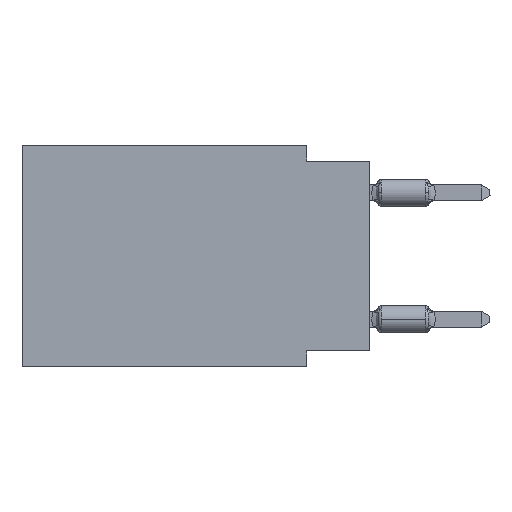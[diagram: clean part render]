
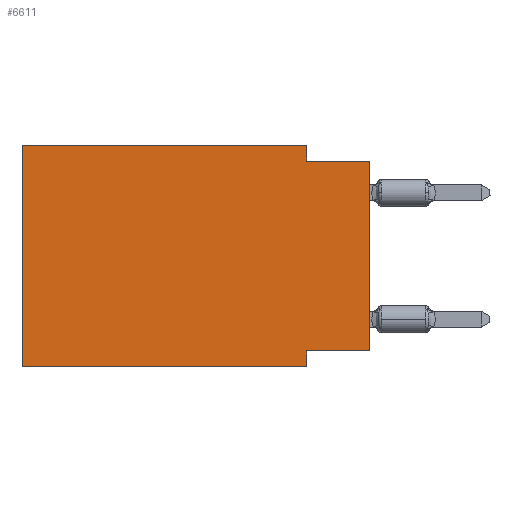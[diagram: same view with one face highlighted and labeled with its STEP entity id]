
A CAD part, left-side view. The second image highlights one B-rep face of the part: STEP entity #6611.
In plain terms, the highlighted planar face has unit normal (-1, 0, 0).
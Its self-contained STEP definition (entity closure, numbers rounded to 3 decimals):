
#25 = VECTOR ( 'NONE', #5033, 1000. ) ;
#152 = ORIENTED_EDGE ( 'NONE', *, *, #23666, .F. ) ;
#1148 = CARTESIAN_POINT ( 'NONE',  ( 0., 13.97, 0. ) ) ;
#2047 = CARTESIAN_POINT ( 'NONE',  ( 0., 13.97, -8.89 ) ) ;
#2530 = ORIENTED_EDGE ( 'NONE', *, *, #20713, .T. ) ;
#3022 = VERTEX_POINT ( 'NONE', #24234 ) ;
#4364 = EDGE_LOOP ( 'NONE', ( #2530, #10978, #5514, #17038, #152, #25755, #10705, #10744 ) ) ;
#4492 = CARTESIAN_POINT ( 'NONE',  ( 0., 13.97, 0. ) ) ;
#4743 = VERTEX_POINT ( 'NONE', #25854 ) ;
#4874 = VERTEX_POINT ( 'NONE', #2047 ) ;
#4876 = EDGE_CURVE ( 'NONE', #5937, #13253, #10589, .T. ) ;
#5033 = DIRECTION ( 'NONE',  ( 0., 0., 1. ) ) ;
#5514 = ORIENTED_EDGE ( 'NONE', *, *, #19162, .F. ) ;
#5937 = VERTEX_POINT ( 'NONE', #9729 ) ;
#6396 = VERTEX_POINT ( 'NONE', #25724 ) ;
#6611 = ADVANCED_FACE ( 'NONE', ( #18299 ), #14349, .F. ) ;
#7750 = EDGE_CURVE ( 'NONE', #8501, #6396, #24331, .T. ) ;
#8501 = VERTEX_POINT ( 'NONE', #12632 ) ;
#9103 = CARTESIAN_POINT ( 'NONE',  ( 0., 0., 0. ) ) ;
#9175 = CARTESIAN_POINT ( 'NONE',  ( 0., 2.54, -8.255 ) ) ;
#9729 = CARTESIAN_POINT ( 'NONE',  ( 0., 0., -8.255 ) ) ;
#10153 = DIRECTION ( 'NONE',  ( 0., 0., -1. ) ) ;
#10405 = DIRECTION ( 'NONE',  ( 0., -1., 0. ) ) ;
#10589 = LINE ( 'NONE', #21653, #26230 ) ;
#10705 = ORIENTED_EDGE ( 'NONE', *, *, #14092, .F. ) ;
#10744 = ORIENTED_EDGE ( 'NONE', *, *, #4876, .F. ) ;
#10776 = DIRECTION ( 'NONE',  ( 0., -1., 0. ) ) ;
#10978 = ORIENTED_EDGE ( 'NONE', *, *, #7750, .F. ) ;
#12194 = EDGE_CURVE ( 'NONE', #4743, #3022, #23680, .T. ) ;
#12384 = CARTESIAN_POINT ( 'NONE',  ( 0., 13.97, 0. ) ) ;
#12632 = CARTESIAN_POINT ( 'NONE',  ( 0., 2.54, -0.635 ) ) ;
#13253 = VERTEX_POINT ( 'NONE', #9175 ) ;
#13336 = VECTOR ( 'NONE', #17233, 1000. ) ;
#13892 = DIRECTION ( 'NONE',  ( 0., 0., 1. ) ) ;
#14092 = EDGE_CURVE ( 'NONE', #13253, #20812, #17506, .T. ) ;
#14349 = PLANE ( 'NONE',  #15550 ) ;
#15550 = AXIS2_PLACEMENT_3D ( 'NONE', #12384, #18711, #10153 ) ;
#17038 = ORIENTED_EDGE ( 'NONE', *, *, #12194, .F. ) ;
#17233 = DIRECTION ( 'NONE',  ( 0., 0., -1. ) ) ;
#17506 = LINE ( 'NONE', #17938, #19445 ) ;
#17897 = DIRECTION ( 'NONE',  ( 0., -1., 0. ) ) ;
#17938 = CARTESIAN_POINT ( 'NONE',  ( 0., 2.54, -8.89 ) ) ;
#18299 = FACE_OUTER_BOUND ( 'NONE', #4364, .T. ) ;
#18711 = DIRECTION ( 'NONE',  ( 1., 0., 0. ) ) ;
#19147 = DIRECTION ( 'NONE',  ( 0., 1., 0. ) ) ;
#19162 = EDGE_CURVE ( 'NONE', #3022, #8501, #21179, .T. ) ;
#19445 = VECTOR ( 'NONE', #19899, 1000. ) ;
#19893 = LINE ( 'NONE', #9103, #25 ) ;
#19899 = DIRECTION ( 'NONE',  ( 0., 0., -1. ) ) ;
#20086 = LINE ( 'NONE', #1148, #24801 ) ;
#20713 = EDGE_CURVE ( 'NONE', #5937, #6396, #19893, .T. ) ;
#20812 = VERTEX_POINT ( 'NONE', #21855 ) ;
#20934 = CARTESIAN_POINT ( 'NONE',  ( 0., 13.97, -8.89 ) ) ;
#21179 = LINE ( 'NONE', #25789, #13336 ) ;
#21208 = VECTOR ( 'NONE', #10405, 1000. ) ;
#21653 = CARTESIAN_POINT ( 'NONE',  ( 0., 0., -8.255 ) ) ;
#21855 = CARTESIAN_POINT ( 'NONE',  ( 0., 2.54, -8.89 ) ) ;
#23666 = EDGE_CURVE ( 'NONE', #4874, #4743, #20086, .T. ) ;
#23680 = LINE ( 'NONE', #4492, #25359 ) ;
#24234 = CARTESIAN_POINT ( 'NONE',  ( 0., 2.54, 0. ) ) ;
#24331 = LINE ( 'NONE', #26564, #26788 ) ;
#24801 = VECTOR ( 'NONE', #13892, 1000. ) ;
#25359 = VECTOR ( 'NONE', #10776, 1000. ) ;
#25724 = CARTESIAN_POINT ( 'NONE',  ( 0., 0., -0.635 ) ) ;
#25755 = ORIENTED_EDGE ( 'NONE', *, *, #26005, .T. ) ;
#25789 = CARTESIAN_POINT ( 'NONE',  ( 0., 2.54, 0. ) ) ;
#25854 = CARTESIAN_POINT ( 'NONE',  ( 0., 13.97, 0. ) ) ;
#26005 = EDGE_CURVE ( 'NONE', #4874, #20812, #27495, .T. ) ;
#26230 = VECTOR ( 'NONE', #19147, 1000. ) ;
#26564 = CARTESIAN_POINT ( 'NONE',  ( 0., 0., -0.635 ) ) ;
#26788 = VECTOR ( 'NONE', #17897, 1000. ) ;
#27495 = LINE ( 'NONE', #20934, #21208 ) ;
